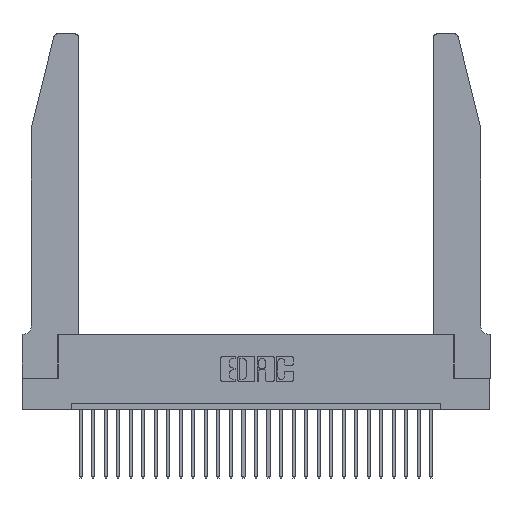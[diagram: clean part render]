
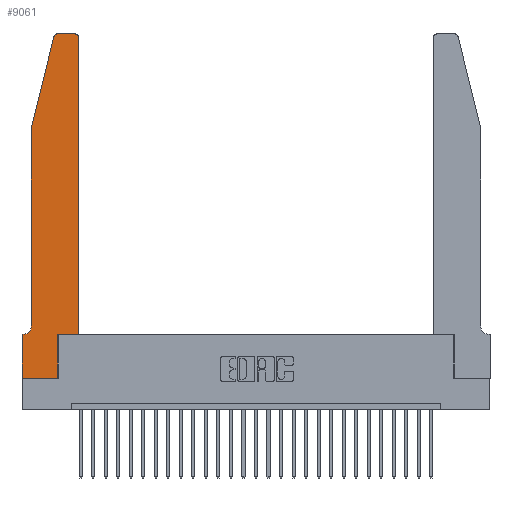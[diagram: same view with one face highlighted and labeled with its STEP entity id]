
A CAD part, top view. The second image highlights one B-rep face of the part: STEP entity #9061.
In plain terms, the highlighted planar face has unit normal (0, 0, 1).
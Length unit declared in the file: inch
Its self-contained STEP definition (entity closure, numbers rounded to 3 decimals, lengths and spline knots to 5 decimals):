
#113 = FACE_OUTER_BOUND ( 'NONE', #24484, .T. ) ;
#192 = LINE ( 'NONE', #20159, #7097 ) ;
#572 = VERTEX_POINT ( 'NONE', #6108 ) ;
#997 = AXIS2_PLACEMENT_3D ( 'NONE', #8240, #27444, #16553 ) ;
#1278 = ORIENTED_EDGE ( 'NONE', *, *, #28123, .T. ) ;
#1609 = CARTESIAN_POINT ( 'NONE',  ( 0.2865, 0., 0.37 ) ) ;
#2487 = CARTESIAN_POINT ( 'NONE',  ( 0., 0., 0.37 ) ) ;
#2615 = DIRECTION ( 'NONE',  ( 0., 1., 0. ) ) ;
#3775 = ORIENTED_EDGE ( 'NONE', *, *, #19469, .T. ) ;
#4003 = LINE ( 'NONE', #17668, #23514 ) ;
#4008 = EDGE_CURVE ( 'NONE', #19743, #12361, #7357, .T. ) ;
#4037 = DIRECTION ( 'NONE',  ( 0., 0., 1. ) ) ;
#4115 = LINE ( 'NONE', #17475, #14397 ) ;
#4218 = CARTESIAN_POINT ( 'NONE',  ( 0., 0., 0.37 ) ) ;
#4519 = CARTESIAN_POINT ( 'NONE',  ( 0.4205, 2.72, 0.37 ) ) ;
#4728 = ORIENTED_EDGE ( 'NONE', *, *, #4008, .T. ) ;
#4861 = CARTESIAN_POINT ( 'NONE',  ( 0.4505, 0.35, 0.37 ) ) ;
#5071 = VERTEX_POINT ( 'NONE', #17232 ) ;
#5214 = EDGE_CURVE ( 'NONE', #17929, #18890, #14056, .T. ) ;
#5396 = ORIENTED_EDGE ( 'NONE', *, *, #14651, .T. ) ;
#5436 = VECTOR ( 'NONE', #5503, 39.37008 ) ;
#5503 = DIRECTION ( 'NONE',  ( -1., 0., 0. ) ) ;
#5555 = ORIENTED_EDGE ( 'NONE', *, *, #22334, .T. ) ;
#5788 = CARTESIAN_POINT ( 'NONE',  ( 0.284, 2.75, 0.37 ) ) ;
#5833 = ORIENTED_EDGE ( 'NONE', *, *, #18762, .T. ) ;
#5880 = ORIENTED_EDGE ( 'NONE', *, *, #5906, .T. ) ;
#5906 = EDGE_CURVE ( 'NONE', #12120, #17929, #7239, .T. ) ;
#6108 = CARTESIAN_POINT ( 'NONE',  ( 0.4205, 2.75, 0.37 ) ) ;
#6136 = AXIS2_PLACEMENT_3D ( 'NONE', #25739, #4037, #17228 ) ;
#6478 = DIRECTION ( 'NONE',  ( 1., 0., 0. ) ) ;
#7097 = VECTOR ( 'NONE', #17689, 39.37008 ) ;
#7239 = LINE ( 'NONE', #11472, #16409 ) ;
#7357 = LINE ( 'NONE', #8994, #16882 ) ;
#7704 = EDGE_CURVE ( 'NONE', #19510, #18182, #19395, .T. ) ;
#8240 = CARTESIAN_POINT ( 'NONE',  ( 0., 0.35, 0.37 ) ) ;
#8252 = VECTOR ( 'NONE', #22091, 39.37008 ) ;
#8254 = AXIS2_PLACEMENT_3D ( 'NONE', #4519, #8945, #19808 ) ;
#8945 = DIRECTION ( 'NONE',  ( 0., 0., 1. ) ) ;
#8994 = CARTESIAN_POINT ( 'NONE',  ( 0.4505, 0.35, 0.37 ) ) ;
#9061 = ADVANCED_FACE ( 'NONE', ( #113 ), #27774, .T. ) ;
#9095 = ORIENTED_EDGE ( 'NONE', *, *, #10509, .T. ) ;
#9126 = CIRCLE ( 'NONE', #21586, 0.07 ) ;
#9811 = ORIENTED_EDGE ( 'NONE', *, *, #7704, .T. ) ;
#10509 = EDGE_CURVE ( 'NONE', #5071, #12120, #22324, .T. ) ;
#11472 = CARTESIAN_POINT ( 'NONE',  ( 0., 0., 0.37 ) ) ;
#12052 = CARTESIAN_POINT ( 'NONE',  ( 0.2605, 2.75, 0.37 ) ) ;
#12120 = VERTEX_POINT ( 'NONE', #18351 ) ;
#12361 = VERTEX_POINT ( 'NONE', #4861 ) ;
#12994 = LINE ( 'NONE', #12052, #5436 ) ;
#13145 = DIRECTION ( 'NONE',  ( -1., 0., 0. ) ) ;
#13276 = DIRECTION ( 'NONE',  ( 0., -1., 0. ) ) ;
#13983 = EDGE_CURVE ( 'NONE', #25048, #15164, #192, .T. ) ;
#14056 = LINE ( 'NONE', #2487, #8252 ) ;
#14397 = VECTOR ( 'NONE', #19762, 39.37008 ) ;
#14651 = EDGE_CURVE ( 'NONE', #15164, #5071, #9126, .T. ) ;
#14712 = ORIENTED_EDGE ( 'NONE', *, *, #5214, .T. ) ;
#15164 = VERTEX_POINT ( 'NONE', #16723 ) ;
#16409 = VECTOR ( 'NONE', #13276, 39.37008 ) ;
#16553 = DIRECTION ( 'NONE',  ( 1., 0., 0. ) ) ;
#16723 = CARTESIAN_POINT ( 'NONE',  ( 0.0755, 0.42, 0.37 ) ) ;
#16784 = VERTEX_POINT ( 'NONE', #25767 ) ;
#16882 = VECTOR ( 'NONE', #6478, 39.37008 ) ;
#17228 = DIRECTION ( 'NONE',  ( 1., 0., 0. ) ) ;
#17232 = CARTESIAN_POINT ( 'NONE',  ( 0.0055, 0.35, 0.37 ) ) ;
#17475 = CARTESIAN_POINT ( 'NONE',  ( 0.2865, 0.35, 0.37 ) ) ;
#17668 = CARTESIAN_POINT ( 'NONE',  ( 0.0755, 2., 0.37 ) ) ;
#17689 = DIRECTION ( 'NONE',  ( 0., -1., 0. ) ) ;
#17878 = CIRCLE ( 'NONE', #8254, 0.03 ) ;
#17929 = VERTEX_POINT ( 'NONE', #4218 ) ;
#17938 = LINE ( 'NONE', #22404, #24055 ) ;
#18182 = VERTEX_POINT ( 'NONE', #27464 ) ;
#18282 = DIRECTION ( 'NONE',  ( 0., 0., -1. ) ) ;
#18351 = CARTESIAN_POINT ( 'NONE',  ( 0., 0.35, 0.37 ) ) ;
#18762 = EDGE_CURVE ( 'NONE', #572, #19510, #12994, .T. ) ;
#18890 = VERTEX_POINT ( 'NONE', #1609 ) ;
#19395 = CIRCLE ( 'NONE', #6136, 0.03 ) ;
#19469 = EDGE_CURVE ( 'NONE', #18182, #25048, #4003, .T. ) ;
#19510 = VERTEX_POINT ( 'NONE', #5788 ) ;
#19743 = VERTEX_POINT ( 'NONE', #27385 ) ;
#19762 = DIRECTION ( 'NONE',  ( 0., 1., 0. ) ) ;
#19808 = DIRECTION ( 'NONE',  ( 1., 0., 0. ) ) ;
#20159 = CARTESIAN_POINT ( 'NONE',  ( 0.0755, 2., 0.37 ) ) ;
#21586 = AXIS2_PLACEMENT_3D ( 'NONE', #24561, #18282, #22472 ) ;
#21818 = EDGE_CURVE ( 'NONE', #12361, #16784, #17938, .T. ) ;
#22091 = DIRECTION ( 'NONE',  ( 1., 0., 0. ) ) ;
#22186 = CARTESIAN_POINT ( 'NONE',  ( 0.0755, 2., 0.37 ) ) ;
#22324 = LINE ( 'NONE', #26211, #23656 ) ;
#22334 = EDGE_CURVE ( 'NONE', #16784, #572, #17878, .T. ) ;
#22404 = CARTESIAN_POINT ( 'NONE',  ( 0.4505, 0.35, 0.37 ) ) ;
#22472 = DIRECTION ( 'NONE',  ( -1., 0., 0. ) ) ;
#22593 = ORIENTED_EDGE ( 'NONE', *, *, #21818, .T. ) ;
#23514 = VECTOR ( 'NONE', #24536, 39.37008 ) ;
#23656 = VECTOR ( 'NONE', #13145, 39.37008 ) ;
#24055 = VECTOR ( 'NONE', #2615, 39.37008 ) ;
#24484 = EDGE_LOOP ( 'NONE', ( #5833, #9811, #3775, #26234, #5396, #9095, #5880, #14712, #1278, #4728, #22593, #5555 ) ) ;
#24536 = DIRECTION ( 'NONE',  ( -0.239, -0.971, 0. ) ) ;
#24561 = CARTESIAN_POINT ( 'NONE',  ( 0.0055, 0.42, 0.37 ) ) ;
#25048 = VERTEX_POINT ( 'NONE', #22186 ) ;
#25739 = CARTESIAN_POINT ( 'NONE',  ( 0.284, 2.72, 0.37 ) ) ;
#25767 = CARTESIAN_POINT ( 'NONE',  ( 0.4505, 2.72, 0.37 ) ) ;
#26211 = CARTESIAN_POINT ( 'NONE',  ( 0.0755, 0.35, 0.37 ) ) ;
#26234 = ORIENTED_EDGE ( 'NONE', *, *, #13983, .T. ) ;
#27385 = CARTESIAN_POINT ( 'NONE',  ( 0.2865, 0.35, 0.37 ) ) ;
#27444 = DIRECTION ( 'NONE',  ( 0., 0., 1. ) ) ;
#27464 = CARTESIAN_POINT ( 'NONE',  ( 0.25487, 2.72718, 0.37 ) ) ;
#27774 = PLANE ( 'NONE',  #997 ) ;
#28123 = EDGE_CURVE ( 'NONE', #18890, #19743, #4115, .T. ) ;
